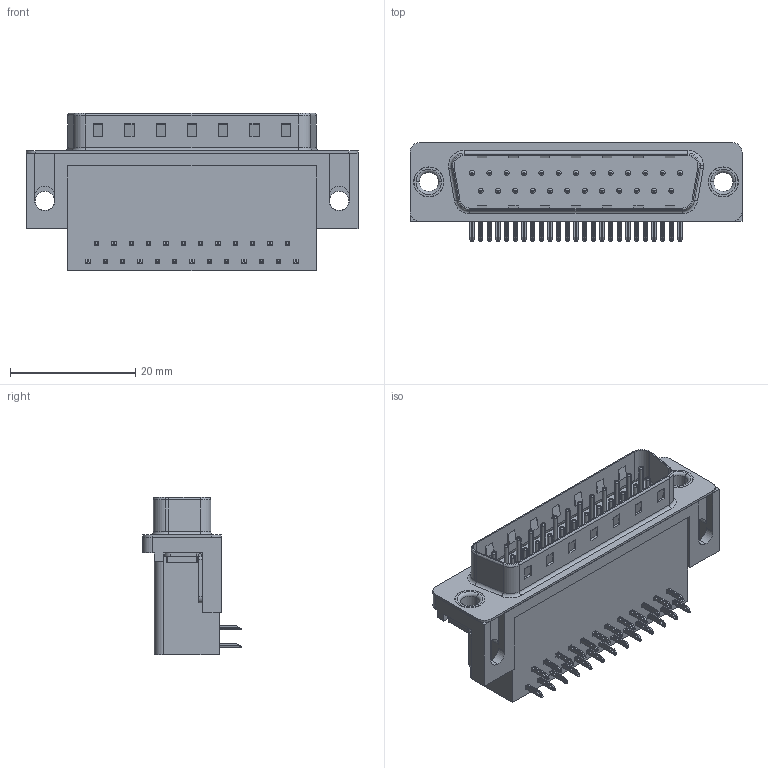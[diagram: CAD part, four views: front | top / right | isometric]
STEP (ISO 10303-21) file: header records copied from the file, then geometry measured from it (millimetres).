
FILE_DESCRIPTION (( 'STEP AP203' ), '1' );
FILE_NAME ('625-025-662-011.STEP', '2018-11-06T03:11:51', ( '' ), ( '' ), 'SwSTEP 2.0', 'SolidWorks 2016', '' );
FILE_SCHEMA (( 'CONFIG_CONTROL_DESIGN' ));
Length unit declared in the file: millimetre
Products named in the file (7): 625-025-662-011; 625 Housing_25 Socket; 625 Shell_25 Socket; 625 Contact Bottom; 625 Contact Top; 625 Thru Hole Board Mount; 625 Thru Hole Rivet
Assembly tree (31 placements, depth 2):
  625-025-662-011
    625 Housing_25 Socket
    625 Shell_25 Socket
    625 Contact Bottom  x12
    625 Contact Top  x13
    625 Thru Hole Board Mount  x2
    625 Thru Hole Rivet  x2
Bounding box: 53.04 x 15.73 x 25.16 mm (x, y, z)
Volume: 9149.7 mm3; surface area: 8825.3 mm2
Topology: 31 solids, 31 shells, 2225 faces, 5501 edges, 3395 vertices
Faces by surface type: plane 1405, cylinder 643, torus 177
Entity records: 20399 total; most frequent: DIRECTION 3344, CARTESIAN_POINT 3294, ORIENTED_EDGE 3166, EDGE_CURVE 1583, LINE 1142, VECTOR 1142, AXIS2_PLACEMENT_3D 1101, VERTEX_POINT 1015
